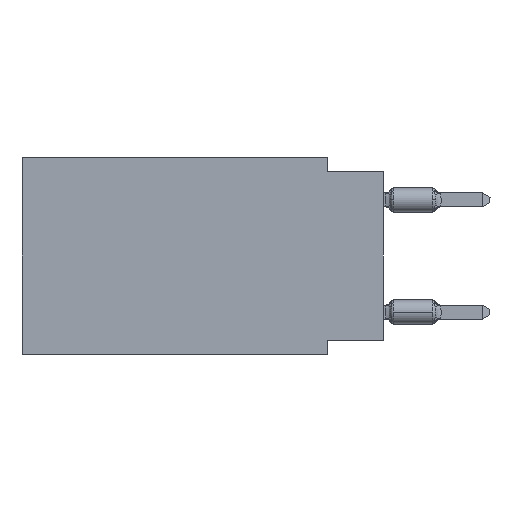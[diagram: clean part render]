
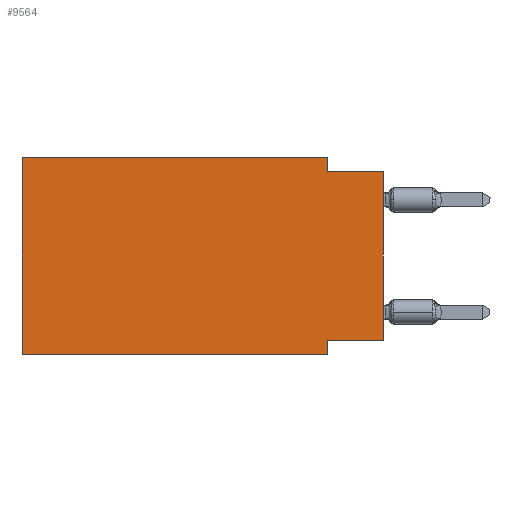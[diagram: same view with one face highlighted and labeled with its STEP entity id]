
A CAD part, left-side view. The second image highlights one B-rep face of the part: STEP entity #9564.
In plain terms, the highlighted planar face has unit normal (-1, 0, 0).
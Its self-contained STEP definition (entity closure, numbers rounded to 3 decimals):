
#1469 = VECTOR ( 'NONE', #5881, 1000. ) ;
#1917 = CARTESIAN_POINT ( 'NONE',  ( 0., 2.54, 0. ) ) ;
#4394 = LINE ( 'NONE', #16252, #24647 ) ;
#5722 = ORIENTED_EDGE ( 'NONE', *, *, #23566, .F. ) ;
#5881 = DIRECTION ( 'NONE',  ( 0., 0., -1. ) ) ;
#8347 = VERTEX_POINT ( 'NONE', #13791 ) ;
#9564 = ADVANCED_FACE ( 'NONE', ( #12258 ), #24630, .F. ) ;
#9583 = EDGE_CURVE ( 'NONE', #40446, #20740, #34065, .T. ) ;
#9809 = CARTESIAN_POINT ( 'NONE',  ( 0., 16.383, 0. ) ) ;
#9849 = EDGE_CURVE ( 'NONE', #20740, #17178, #35889, .T. ) ;
#11570 = CARTESIAN_POINT ( 'NONE',  ( 0., 2.54, -8.89 ) ) ;
#12258 = FACE_OUTER_BOUND ( 'NONE', #41773, .T. ) ;
#13191 = CARTESIAN_POINT ( 'NONE',  ( 0., 16.383, 0. ) ) ;
#13791 = CARTESIAN_POINT ( 'NONE',  ( 0., 16.383, -8.89 ) ) ;
#16127 = DIRECTION ( 'NONE',  ( 0., -1., 0. ) ) ;
#16252 = CARTESIAN_POINT ( 'NONE',  ( 0., 0., 0. ) ) ;
#17178 = VERTEX_POINT ( 'NONE', #45163 ) ;
#18477 = LINE ( 'NONE', #41927, #34386 ) ;
#18512 = CARTESIAN_POINT ( 'NONE',  ( 0., 2.54, -8.89 ) ) ;
#18602 = VECTOR ( 'NONE', #41716, 1000. ) ;
#19573 = CARTESIAN_POINT ( 'NONE',  ( 0., 16.383, 0. ) ) ;
#20245 = EDGE_CURVE ( 'NONE', #47912, #17178, #4394, .T. ) ;
#20740 = VERTEX_POINT ( 'NONE', #33272 ) ;
#20812 = ORIENTED_EDGE ( 'NONE', *, *, #48388, .T. ) ;
#21409 = ORIENTED_EDGE ( 'NONE', *, *, #22292, .F. ) ;
#21951 = DIRECTION ( 'NONE',  ( 0., 0., -1. ) ) ;
#22292 = EDGE_CURVE ( 'NONE', #42035, #40446, #36660, .T. ) ;
#23566 = EDGE_CURVE ( 'NONE', #47912, #51676, #18477, .T. ) ;
#24000 = CARTESIAN_POINT ( 'NONE',  ( 0., 2.54, -8.255 ) ) ;
#24044 = DIRECTION ( 'NONE',  ( 0., -1., 0. ) ) ;
#24630 = PLANE ( 'NONE',  #29304 ) ;
#24647 = VECTOR ( 'NONE', #35741, 1000. ) ;
#25406 = DIRECTION ( 'NONE',  ( 1., 0., 0. ) ) ;
#27210 = EDGE_CURVE ( 'NONE', #8347, #42035, #41426, .T. ) ;
#27734 = CARTESIAN_POINT ( 'NONE',  ( 0., 0., -0.635 ) ) ;
#27828 = VERTEX_POINT ( 'NONE', #11570 ) ;
#29304 = AXIS2_PLACEMENT_3D ( 'NONE', #48900, #25406, #21951 ) ;
#30966 = EDGE_CURVE ( 'NONE', #51676, #27828, #50179, .T. ) ;
#30974 = ORIENTED_EDGE ( 'NONE', *, *, #9849, .F. ) ;
#31871 = VECTOR ( 'NONE', #24044, 1000. ) ;
#32901 = VECTOR ( 'NONE', #16127, 1000. ) ;
#33272 = CARTESIAN_POINT ( 'NONE',  ( 0., 2.54, -0.635 ) ) ;
#34033 = DIRECTION ( 'NONE',  ( 0., 0., 1. ) ) ;
#34065 = LINE ( 'NONE', #1917, #1469 ) ;
#34273 = CARTESIAN_POINT ( 'NONE',  ( 0., 2.54, 0. ) ) ;
#34386 = VECTOR ( 'NONE', #34558, 1000. ) ;
#34558 = DIRECTION ( 'NONE',  ( 0., 1., 0. ) ) ;
#35741 = DIRECTION ( 'NONE',  ( 0., 0., 1. ) ) ;
#35889 = LINE ( 'NONE', #27734, #31871 ) ;
#36187 = CARTESIAN_POINT ( 'NONE',  ( 0., 0., -8.255 ) ) ;
#36660 = LINE ( 'NONE', #19573, #38689 ) ;
#37358 = ORIENTED_EDGE ( 'NONE', *, *, #27210, .F. ) ;
#38689 = VECTOR ( 'NONE', #48568, 1000. ) ;
#40446 = VERTEX_POINT ( 'NONE', #34273 ) ;
#41426 = LINE ( 'NONE', #9809, #50527 ) ;
#41716 = DIRECTION ( 'NONE',  ( 0., 0., -1. ) ) ;
#41773 = EDGE_LOOP ( 'NONE', ( #47742, #30974, #42296, #21409, #37358, #20812, #45183, #5722 ) ) ;
#41927 = CARTESIAN_POINT ( 'NONE',  ( 0., 0., -8.255 ) ) ;
#42035 = VERTEX_POINT ( 'NONE', #13191 ) ;
#42296 = ORIENTED_EDGE ( 'NONE', *, *, #9583, .F. ) ;
#45163 = CARTESIAN_POINT ( 'NONE',  ( 0., 0., -0.635 ) ) ;
#45183 = ORIENTED_EDGE ( 'NONE', *, *, #30966, .F. ) ;
#47742 = ORIENTED_EDGE ( 'NONE', *, *, #20245, .T. ) ;
#47912 = VERTEX_POINT ( 'NONE', #36187 ) ;
#48388 = EDGE_CURVE ( 'NONE', #8347, #27828, #49069, .T. ) ;
#48568 = DIRECTION ( 'NONE',  ( 0., -1., 0. ) ) ;
#48802 = CARTESIAN_POINT ( 'NONE',  ( 0., 16.383, -8.89 ) ) ;
#48900 = CARTESIAN_POINT ( 'NONE',  ( 0., 16.383, 0. ) ) ;
#49069 = LINE ( 'NONE', #48802, #32901 ) ;
#50179 = LINE ( 'NONE', #18512, #18602 ) ;
#50527 = VECTOR ( 'NONE', #34033, 1000. ) ;
#51676 = VERTEX_POINT ( 'NONE', #24000 ) ;
